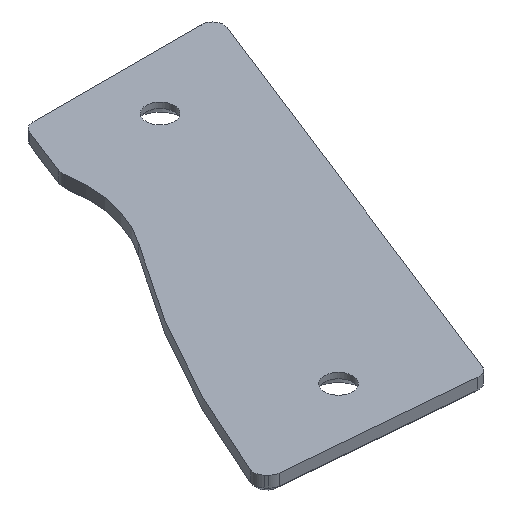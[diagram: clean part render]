
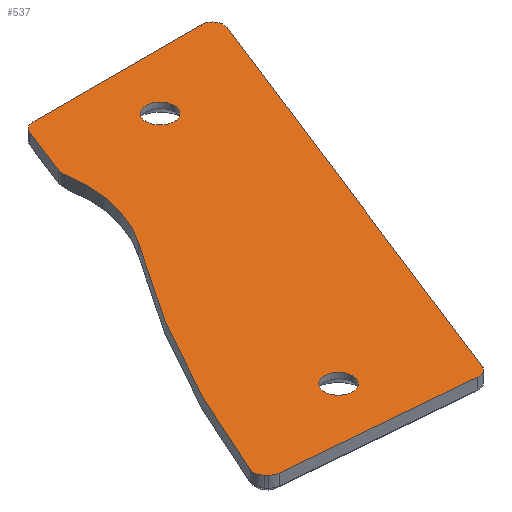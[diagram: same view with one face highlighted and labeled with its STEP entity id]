
A CAD part, isometric view. The second image highlights one B-rep face of the part: STEP entity #537.
In plain terms, the highlighted planar face has unit normal (0, 0, 1).
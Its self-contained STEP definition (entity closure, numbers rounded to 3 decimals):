
#17=FACE_BOUND('',#105,.T.);
#18=FACE_BOUND('',#106,.T.);
#40=PLANE('',#613);
#70=FACE_OUTER_BOUND('',#104,.T.);
#104=EDGE_LOOP('',(#475,#476,#477,#478,#479,#480,#481,#482,#483,#484,#485,
#486,#487));
#105=EDGE_LOOP('',(#488));
#106=EDGE_LOOP('',(#489));
#135=LINE('',#877,#179);
#138=LINE('',#885,#182);
#147=LINE('',#920,#191);
#148=LINE('',#922,#192);
#149=LINE('',#924,#193);
#179=VECTOR('',#707,10.);
#182=VECTOR('',#716,10.);
#191=VECTOR('',#757,10.);
#192=VECTOR('',#760,10.);
#193=VECTOR('',#763,10.);
#214=CIRCLE('',#584,2.);
#215=CIRCLE('',#587,2.);
#216=CIRCLE('',#590,2.);
#217=CIRCLE('',#592,22.992);
#218=CIRCLE('',#594,205.75);
#221=CIRCLE('',#599,2.);
#222=CIRCLE('',#601,2.);
#223=CIRCLE('',#603,2.);
#224=CIRCLE('',#608,2.5);
#226=CIRCLE('',#611,2.5);
#254=VERTEX_POINT('',#869);
#255=VERTEX_POINT('',#871);
#256=VERTEX_POINT('',#875);
#257=VERTEX_POINT('',#879);
#258=VERTEX_POINT('',#883);
#259=VERTEX_POINT('',#887);
#260=VERTEX_POINT('',#891);
#261=VERTEX_POINT('',#895);
#264=VERTEX_POINT('',#904);
#265=VERTEX_POINT('',#906);
#266=VERTEX_POINT('',#910);
#267=VERTEX_POINT('',#912);
#268=VERTEX_POINT('',#916);
#269=VERTEX_POINT('',#926);
#271=VERTEX_POINT('',#932);
#313=EDGE_CURVE('',#255,#254,#214,.T.);
#316=EDGE_CURVE('',#254,#256,#135,.T.);
#318=EDGE_CURVE('',#256,#257,#215,.T.);
#320=EDGE_CURVE('',#257,#258,#138,.T.);
#322=EDGE_CURVE('',#258,#259,#216,.T.);
#324=EDGE_CURVE('',#259,#260,#217,.T.);
#326=EDGE_CURVE('',#260,#261,#218,.T.);
#330=EDGE_CURVE('',#265,#264,#221,.T.);
#333=EDGE_CURVE('',#267,#266,#222,.T.);
#336=EDGE_CURVE('',#261,#268,#223,.T.);
#337=EDGE_CURVE('',#268,#265,#147,.T.);
#338=EDGE_CURVE('',#264,#267,#148,.T.);
#339=EDGE_CURVE('',#266,#255,#149,.T.);
#340=EDGE_CURVE('',#269,#269,#224,.T.);
#343=EDGE_CURVE('',#271,#271,#226,.T.);
#475=ORIENTED_EDGE('',*,*,#330,.T.);
#476=ORIENTED_EDGE('',*,*,#338,.T.);
#477=ORIENTED_EDGE('',*,*,#333,.T.);
#478=ORIENTED_EDGE('',*,*,#339,.T.);
#479=ORIENTED_EDGE('',*,*,#313,.T.);
#480=ORIENTED_EDGE('',*,*,#316,.T.);
#481=ORIENTED_EDGE('',*,*,#318,.T.);
#482=ORIENTED_EDGE('',*,*,#320,.T.);
#483=ORIENTED_EDGE('',*,*,#322,.T.);
#484=ORIENTED_EDGE('',*,*,#324,.T.);
#485=ORIENTED_EDGE('',*,*,#326,.T.);
#486=ORIENTED_EDGE('',*,*,#336,.T.);
#487=ORIENTED_EDGE('',*,*,#337,.T.);
#488=ORIENTED_EDGE('',*,*,#343,.T.);
#489=ORIENTED_EDGE('',*,*,#340,.T.);
#537=ADVANCED_FACE('',(#70,#17,#18),#40,.F.);
#584=AXIS2_PLACEMENT_3D('',#872,#701,#702);
#587=AXIS2_PLACEMENT_3D('',#881,#711,#712);
#590=AXIS2_PLACEMENT_3D('',#889,#720,#721);
#592=AXIS2_PLACEMENT_3D('',#893,#725,#726);
#594=AXIS2_PLACEMENT_3D('',#897,#730,#731);
#599=AXIS2_PLACEMENT_3D('',#907,#741,#742);
#601=AXIS2_PLACEMENT_3D('',#913,#747,#748);
#603=AXIS2_PLACEMENT_3D('',#918,#753,#754);
#608=AXIS2_PLACEMENT_3D('',#927,#766,#767);
#611=AXIS2_PLACEMENT_3D('',#933,#773,#774);
#613=AXIS2_PLACEMENT_3D('',#937,#778,#779);
#701=DIRECTION('center_axis',(0.,0.,1.));
#702=DIRECTION('ref_axis',(0.827,0.563,0.));
#707=DIRECTION('',(-1.,0.,0.));
#711=DIRECTION('center_axis',(0.,0.,1.));
#712=DIRECTION('ref_axis',(-0.563,0.827,0.));
#716=DIRECTION('',(-0.367,-0.93,0.));
#720=DIRECTION('center_axis',(0.,0.,1.));
#721=DIRECTION('ref_axis',(-0.995,0.103,0.));
#725=DIRECTION('center_axis',(0.,0.,-1.));
#726=DIRECTION('ref_axis',(0.98,0.2,0.));
#730=DIRECTION('center_axis',(0.,0.,1.));
#731=DIRECTION('ref_axis',(-0.93,0.367,0.));
#741=DIRECTION('center_axis',(0.,0.,1.));
#742=DIRECTION('ref_axis',(-0.432,-0.902,0.));
#747=DIRECTION('center_axis',(0.,0.,1.));
#748=DIRECTION('ref_axis',(0.525,-0.851,0.));
#753=DIRECTION('center_axis',(0.,0.,1.));
#754=DIRECTION('ref_axis',(-0.982,-0.191,0.));
#757=DIRECTION('',(0.694,-0.72,0.));
#760=DIRECTION('',(0.996,-0.089,0.));
#763=DIRECTION('',(0.367,0.93,0.));
#766=DIRECTION('center_axis',(0.,0.,-1.));
#767=DIRECTION('ref_axis',(-1.,0.,0.));
#773=DIRECTION('center_axis',(0.,0.,-1.));
#774=DIRECTION('ref_axis',(-1.,0.,0.));
#778=DIRECTION('center_axis',(0.,0.,-1.));
#779=DIRECTION('ref_axis',(1.,0.,0.));
#869=CARTESIAN_POINT('',(60.539,-13.063,-13.9));
#871=CARTESIAN_POINT('',(62.4,-15.796,-13.9));
#872=CARTESIAN_POINT('Origin',(60.539,-15.063,-13.9));
#875=CARTESIAN_POINT('',(30.503,-13.063,-13.9));
#877=CARTESIAN_POINT('',(34.353,-13.063,-13.9));
#879=CARTESIAN_POINT('',(28.642,-14.33,-13.9));
#881=CARTESIAN_POINT('Origin',(30.503,-15.063,-13.9));
#883=CARTESIAN_POINT('',(25.267,-22.899,-13.9));
#885=CARTESIAN_POINT('',(21.859,-31.55,-13.9));
#887=CARTESIAN_POINT('',(25.156,-23.967,-13.9));
#889=CARTESIAN_POINT('Origin',(27.128,-23.632,-13.9));
#891=CARTESIAN_POINT('',(21.093,-41.331,-13.9));
#893=CARTESIAN_POINT('Origin',(2.489,-27.821,-13.9));
#895=CARTESIAN_POINT('',(-3.847,-86.164,-13.9));
#897=CARTESIAN_POINT('Origin',(187.022,-162.989,-13.9));
#904=CARTESIAN_POINT('',(-1.796,-89.29,-13.9));
#906=CARTESIAN_POINT('',(-3.058,-88.686,-13.9));
#907=CARTESIAN_POINT('Origin',(-1.618,-87.298,-13.9));
#910=CARTESIAN_POINT('',(32.8,-90.939,-13.9));
#912=CARTESIAN_POINT('',(30.762,-92.198,-13.9));
#913=CARTESIAN_POINT('Origin',(30.94,-90.206,-13.9));
#916=CARTESIAN_POINT('',(-3.432,-88.298,-13.9));
#918=CARTESIAN_POINT('Origin',(-1.992,-86.91,-13.9));
#920=CARTESIAN_POINT('',(-3.181,-88.558,-13.9));
#922=CARTESIAN_POINT('',(32.679,-92.369,-13.9));
#924=CARTESIAN_POINT('',(55.337,-33.725,-13.9));
#926=CARTESIAN_POINT('',(45.632,-23.118,-13.9));
#927=CARTESIAN_POINT('Origin',(43.132,-23.118,-13.9));
#932=CARTESIAN_POINT('',(19.792,-80.791,-13.9));
#933=CARTESIAN_POINT('Origin',(17.292,-80.791,-13.9));
#937=CARTESIAN_POINT('Origin',(38.373,-48.148,-13.9));
